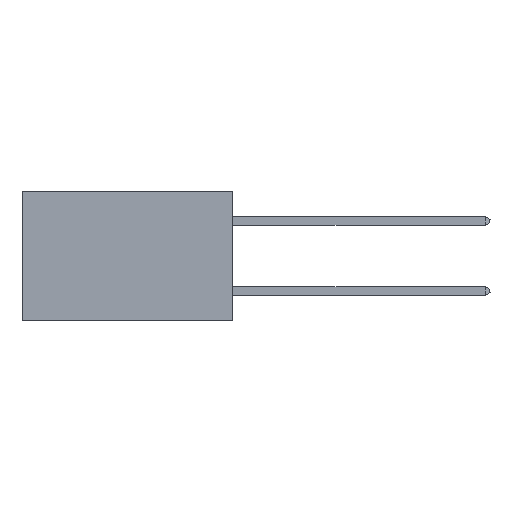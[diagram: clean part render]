
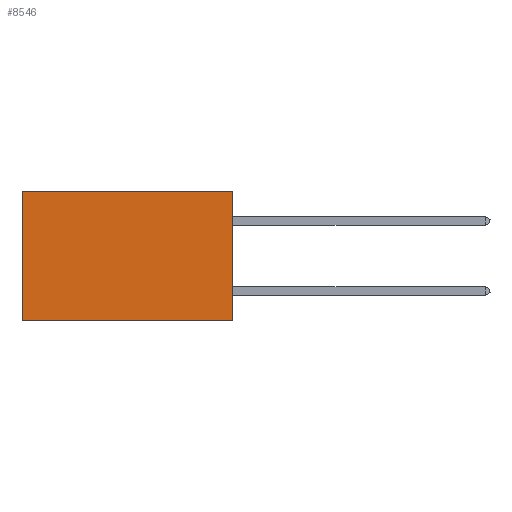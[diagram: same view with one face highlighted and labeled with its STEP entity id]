
A CAD part, left-side view. The second image highlights one B-rep face of the part: STEP entity #8546.
In plain terms, the highlighted planar face has unit normal (-1, 0, 0).
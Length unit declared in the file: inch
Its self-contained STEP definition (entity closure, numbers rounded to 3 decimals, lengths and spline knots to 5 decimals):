
#370 = EDGE_CURVE ( 'NONE', #8521, #39042, #37153, .T. ) ;
#614 = DIRECTION ( 'NONE',  ( 0., 0., -1. ) ) ;
#1612 = FACE_OUTER_BOUND ( 'NONE', #44319, .T. ) ;
#3055 = DIRECTION ( 'NONE',  ( 0., 1., 0. ) ) ;
#3354 = LINE ( 'NONE', #21701, #9380 ) ;
#5192 = CARTESIAN_POINT ( 'NONE',  ( 0.2875, 0., 0. ) ) ;
#5345 = ORIENTED_EDGE ( 'NONE', *, *, #24810, .T. ) ;
#6068 = LINE ( 'NONE', #40001, #45114 ) ;
#6209 = CARTESIAN_POINT ( 'NONE',  ( 0.2875, 0.6, 0. ) ) ;
#8299 = DIRECTION ( 'NONE',  ( 0., 0., -1. ) ) ;
#8521 = VERTEX_POINT ( 'NONE', #39672 ) ;
#8546 = ADVANCED_FACE ( 'NONE', ( #1612 ), #25659, .F. ) ;
#8548 = DIRECTION ( 'NONE',  ( 0., 1., 0. ) ) ;
#9380 = VECTOR ( 'NONE', #614, 39.37008 ) ;
#9627 = VECTOR ( 'NONE', #3055, 39.37008 ) ;
#10776 = VERTEX_POINT ( 'NONE', #6209 ) ;
#14237 = ORIENTED_EDGE ( 'NONE', *, *, #40327, .F. ) ;
#15210 = EDGE_CURVE ( 'NONE', #25781, #10776, #20046, .T. ) ;
#15229 = DIRECTION ( 'NONE',  ( 0., 0., -1. ) ) ;
#18622 = CARTESIAN_POINT ( 'NONE',  ( 0.2875, 0., 0. ) ) ;
#19373 = ORIENTED_EDGE ( 'NONE', *, *, #15210, .T. ) ;
#19629 = CARTESIAN_POINT ( 'NONE',  ( 0.2875, 0., 0. ) ) ;
#20046 = LINE ( 'NONE', #5192, #29395 ) ;
#21701 = CARTESIAN_POINT ( 'NONE',  ( 0.2875, 0., 0. ) ) ;
#24810 = EDGE_CURVE ( 'NONE', #10776, #39042, #6068, .T. ) ;
#25422 = ORIENTED_EDGE ( 'NONE', *, *, #370, .F. ) ;
#25659 = PLANE ( 'NONE',  #31486 ) ;
#25781 = VERTEX_POINT ( 'NONE', #19629 ) ;
#29395 = VECTOR ( 'NONE', #8548, 39.37008 ) ;
#31486 = AXIS2_PLACEMENT_3D ( 'NONE', #18622, #35942, #15229 ) ;
#35942 = DIRECTION ( 'NONE',  ( 1., 0., 0. ) ) ;
#37153 = LINE ( 'NONE', #37955, #9627 ) ;
#37955 = CARTESIAN_POINT ( 'NONE',  ( 0.2875, 0., -0.37 ) ) ;
#39042 = VERTEX_POINT ( 'NONE', #40351 ) ;
#39672 = CARTESIAN_POINT ( 'NONE',  ( 0.2875, 0., -0.37 ) ) ;
#40001 = CARTESIAN_POINT ( 'NONE',  ( 0.2875, 0.6, 0. ) ) ;
#40327 = EDGE_CURVE ( 'NONE', #25781, #8521, #3354, .T. ) ;
#40351 = CARTESIAN_POINT ( 'NONE',  ( 0.2875, 0.6, -0.37 ) ) ;
#44319 = EDGE_LOOP ( 'NONE', ( #5345, #25422, #14237, #19373 ) ) ;
#45114 = VECTOR ( 'NONE', #8299, 39.37008 ) ;
